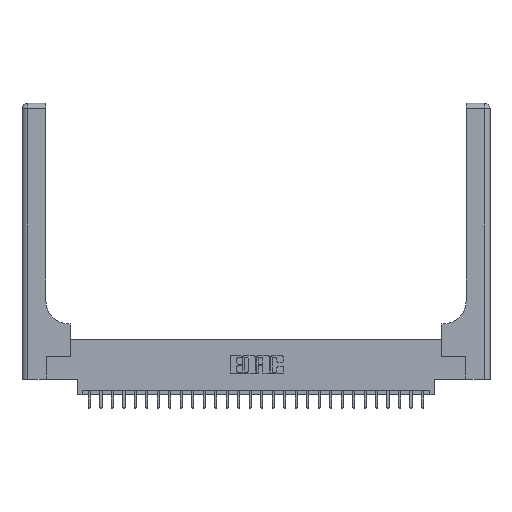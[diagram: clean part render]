
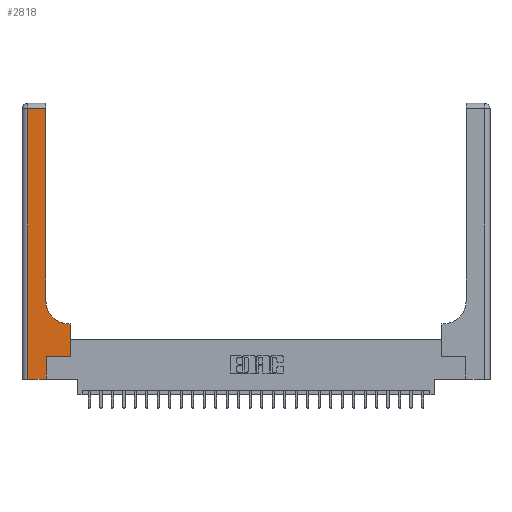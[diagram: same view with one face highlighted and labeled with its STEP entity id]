
A CAD part, top view. The second image highlights one B-rep face of the part: STEP entity #2818.
In plain terms, the highlighted planar face has unit normal (0, 0, 1).
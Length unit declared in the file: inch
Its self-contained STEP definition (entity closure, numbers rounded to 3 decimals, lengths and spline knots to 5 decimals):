
#162 = VERTEX_POINT ( 'NONE', #13662 ) ;
#1104 = EDGE_CURVE ( 'NONE', #11845, #24951, #24765, .T. ) ;
#1358 = EDGE_CURVE ( 'NONE', #14320, #10874, #14987, .T. ) ;
#1412 = DIRECTION ( 'NONE',  ( 0., -1., 0. ) ) ;
#1470 = CARTESIAN_POINT ( 'NONE',  ( 0.26, 2.94, 0.37 ) ) ;
#2008 = VERTEX_POINT ( 'NONE', #1470 ) ;
#2354 = EDGE_CURVE ( 'NONE', #162, #2008, #10113, .T. ) ;
#2555 = EDGE_CURVE ( 'NONE', #5715, #162, #4890, .T. ) ;
#2818 = ADVANCED_FACE ( 'NONE', ( #13141 ), #21342, .F. ) ;
#3072 = CARTESIAN_POINT ( 'NONE',  ( 0.51, 0.85, 0.37 ) ) ;
#3126 = CARTESIAN_POINT ( 'NONE',  ( 0.528, 0.25, 0.37 ) ) ;
#3129 = DIRECTION ( 'NONE',  ( 0., 1., 0. ) ) ;
#3650 = VECTOR ( 'NONE', #4805, 39.37008 ) ;
#4221 = DIRECTION ( 'NONE',  ( 1., 0., 0. ) ) ;
#4774 = ORIENTED_EDGE ( 'NONE', *, *, #18252, .T. ) ;
#4805 = DIRECTION ( 'NONE',  ( 0., 1., 0. ) ) ;
#4890 = CIRCLE ( 'NONE', #25969, 0.25 ) ;
#5194 = DIRECTION ( 'NONE',  ( 1., 0., 0. ) ) ;
#5264 = EDGE_CURVE ( 'NONE', #24951, #15406, #25661, .T. ) ;
#5308 = EDGE_CURVE ( 'NONE', #15406, #13955, #8843, .T. ) ;
#5592 = CARTESIAN_POINT ( 'NONE',  ( 0., 2.94, 0.37 ) ) ;
#5715 = VERTEX_POINT ( 'NONE', #24248 ) ;
#6490 = ORIENTED_EDGE ( 'NONE', *, *, #10715, .T. ) ;
#6731 = ORIENTED_EDGE ( 'NONE', *, *, #26202, .T. ) ;
#8312 = LINE ( 'NONE', #5592, #13803 ) ;
#8843 = LINE ( 'NONE', #13514, #13690 ) ;
#8872 = VECTOR ( 'NONE', #1412, 39.37008 ) ;
#9007 = CARTESIAN_POINT ( 'NONE',  ( 0.265, 0., 0.37 ) ) ;
#9259 = CARTESIAN_POINT ( 'NONE',  ( 0.265, 0.25, 0.37 ) ) ;
#9553 = LINE ( 'NONE', #22588, #25098 ) ;
#9760 = ORIENTED_EDGE ( 'NONE', *, *, #5308, .T. ) ;
#9823 = LINE ( 'NONE', #22979, #15936 ) ;
#10113 = LINE ( 'NONE', #10690, #14317 ) ;
#10690 = CARTESIAN_POINT ( 'NONE',  ( 0.26, 3., 0.37 ) ) ;
#10715 = EDGE_CURVE ( 'NONE', #13955, #5715, #9823, .T. ) ;
#10830 = DIRECTION ( 'NONE',  ( -1., 0., 0. ) ) ;
#10874 = VERTEX_POINT ( 'NONE', #17418 ) ;
#11201 = CARTESIAN_POINT ( 'NONE',  ( 0., 3., 0.37 ) ) ;
#11355 = ORIENTED_EDGE ( 'NONE', *, *, #1104, .T. ) ;
#11845 = VERTEX_POINT ( 'NONE', #17038 ) ;
#13141 = FACE_OUTER_BOUND ( 'NONE', #26320, .T. ) ;
#13238 = ORIENTED_EDGE ( 'NONE', *, *, #2555, .T. ) ;
#13275 = DIRECTION ( 'NONE',  ( -1., 0., 0. ) ) ;
#13514 = CARTESIAN_POINT ( 'NONE',  ( 0.528, 0.25, 0.37 ) ) ;
#13662 = CARTESIAN_POINT ( 'NONE',  ( 0.26, 0.85, 0.37 ) ) ;
#13690 = VECTOR ( 'NONE', #3129, 39.37008 ) ;
#13803 = VECTOR ( 'NONE', #19970, 39.37008 ) ;
#13955 = VERTEX_POINT ( 'NONE', #18089 ) ;
#14317 = VECTOR ( 'NONE', #24753, 39.37008 ) ;
#14320 = VERTEX_POINT ( 'NONE', #17098 ) ;
#14987 = LINE ( 'NONE', #22025, #8872 ) ;
#15406 = VERTEX_POINT ( 'NONE', #3126 ) ;
#15936 = VECTOR ( 'NONE', #10830, 39.37008 ) ;
#17038 = CARTESIAN_POINT ( 'NONE',  ( 0.265, 0., 0.37 ) ) ;
#17098 = CARTESIAN_POINT ( 'NONE',  ( 0.06, 2.94, 0.37 ) ) ;
#17418 = CARTESIAN_POINT ( 'NONE',  ( 0.06, 0., 0.37 ) ) ;
#17541 = DIRECTION ( 'NONE',  ( 0., 0., -1. ) ) ;
#18089 = CARTESIAN_POINT ( 'NONE',  ( 0.528, 0.6, 0.37 ) ) ;
#18252 = EDGE_CURVE ( 'NONE', #10874, #11845, #9553, .T. ) ;
#19941 = CARTESIAN_POINT ( 'NONE',  ( 0.265, 0.25, 0.37 ) ) ;
#19970 = DIRECTION ( 'NONE',  ( -1., 0., 0. ) ) ;
#20360 = VECTOR ( 'NONE', #21494, 39.37008 ) ;
#21285 = ORIENTED_EDGE ( 'NONE', *, *, #1358, .T. ) ;
#21342 = PLANE ( 'NONE',  #24126 ) ;
#21494 = DIRECTION ( 'NONE',  ( 1., 0., 0. ) ) ;
#22025 = CARTESIAN_POINT ( 'NONE',  ( 0.06, 3., 0.37 ) ) ;
#22588 = CARTESIAN_POINT ( 'NONE',  ( 0., 0., 0.37 ) ) ;
#22979 = CARTESIAN_POINT ( 'NONE',  ( 0.26, 0.6, 0.37 ) ) ;
#24126 = AXIS2_PLACEMENT_3D ( 'NONE', #11201, #25334, #13275 ) ;
#24248 = CARTESIAN_POINT ( 'NONE',  ( 0.51, 0.6, 0.37 ) ) ;
#24753 = DIRECTION ( 'NONE',  ( 0., 1., 0. ) ) ;
#24765 = LINE ( 'NONE', #9007, #3650 ) ;
#24880 = ORIENTED_EDGE ( 'NONE', *, *, #5264, .T. ) ;
#24951 = VERTEX_POINT ( 'NONE', #19941 ) ;
#25098 = VECTOR ( 'NONE', #4221, 39.37008 ) ;
#25334 = DIRECTION ( 'NONE',  ( 0., 0., -1. ) ) ;
#25661 = LINE ( 'NONE', #9259, #20360 ) ;
#25969 = AXIS2_PLACEMENT_3D ( 'NONE', #3072, #17541, #5194 ) ;
#26012 = ORIENTED_EDGE ( 'NONE', *, *, #2354, .T. ) ;
#26202 = EDGE_CURVE ( 'NONE', #2008, #14320, #8312, .T. ) ;
#26320 = EDGE_LOOP ( 'NONE', ( #26012, #6731, #21285, #4774, #11355, #24880, #9760, #6490, #13238 ) ) ;
